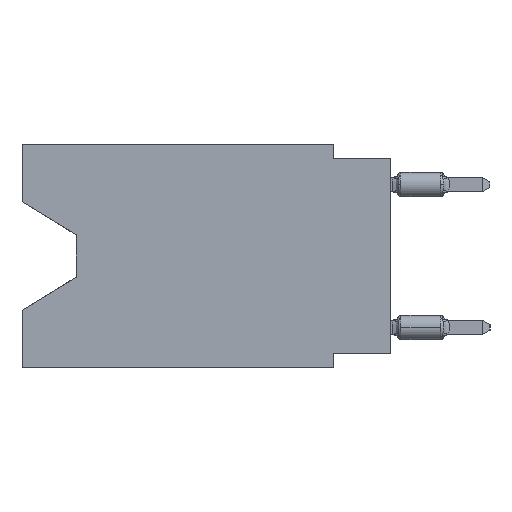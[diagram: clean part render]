
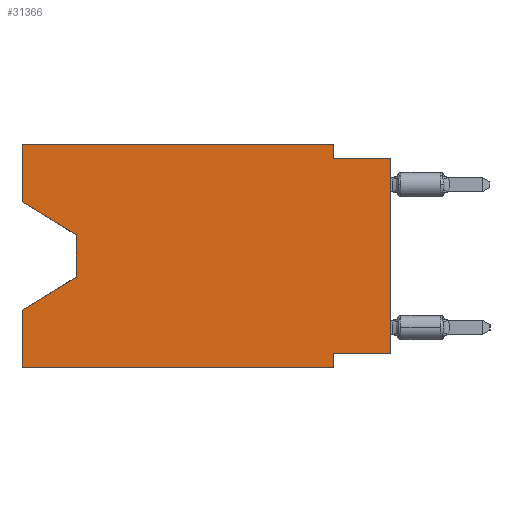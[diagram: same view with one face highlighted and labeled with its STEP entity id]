
A CAD part, left-side view. The second image highlights one B-rep face of the part: STEP entity #31366.
In plain terms, the highlighted planar face has unit normal (-1, 0, 0).
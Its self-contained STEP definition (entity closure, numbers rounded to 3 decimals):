
#161 = VECTOR ( 'NONE', #16425, 1000. ) ;
#222 = DIRECTION ( 'NONE',  ( 0., -1., 0. ) ) ;
#877 = DIRECTION ( 'NONE',  ( 1., 0., 0. ) ) ;
#1106 = CARTESIAN_POINT ( 'NONE',  ( 0., 0., 0. ) ) ;
#1310 = FACE_OUTER_BOUND ( 'NONE', #26498, .T. ) ;
#3058 = EDGE_CURVE ( 'NONE', #6481, #8237, #25895, .T. ) ;
#4183 = DIRECTION ( 'NONE',  ( 0., -1., 0. ) ) ;
#5166 = VERTEX_POINT ( 'NONE', #12029 ) ;
#5691 = EDGE_CURVE ( 'NONE', #41053, #5166, #32945, .T. ) ;
#6027 = CARTESIAN_POINT ( 'NONE',  ( 0., 0., -9.271 ) ) ;
#6143 = CARTESIAN_POINT ( 'NONE',  ( 0., 13.97, -4.013 ) ) ;
#6481 = VERTEX_POINT ( 'NONE', #13730 ) ;
#6867 = LINE ( 'NONE', #6027, #29017 ) ;
#7112 = ORIENTED_EDGE ( 'NONE', *, *, #29976, .F. ) ;
#7142 = VECTOR ( 'NONE', #25878, 1000. ) ;
#7175 = LINE ( 'NONE', #42387, #161 ) ;
#7408 = EDGE_CURVE ( 'NONE', #25848, #33804, #36129, .T. ) ;
#8237 = VERTEX_POINT ( 'NONE', #36243 ) ;
#8855 = ORIENTED_EDGE ( 'NONE', *, *, #14821, .T. ) ;
#8907 = VERTEX_POINT ( 'NONE', #16260 ) ;
#9576 = CARTESIAN_POINT ( 'NONE',  ( 0., 16.383, 0. ) ) ;
#9677 = CARTESIAN_POINT ( 'NONE',  ( 0., 2.54, -9.906 ) ) ;
#9739 = VECTOR ( 'NONE', #33322, 1000. ) ;
#9964 = CARTESIAN_POINT ( 'NONE',  ( 0., 16.383, -9.906 ) ) ;
#10589 = LINE ( 'NONE', #9964, #27923 ) ;
#11843 = DIRECTION ( 'NONE',  ( 0., -0.855, -0.519 ) ) ;
#11880 = CARTESIAN_POINT ( 'NONE',  ( 0., 13.97, -4.013 ) ) ;
#12029 = CARTESIAN_POINT ( 'NONE',  ( 0., 0., -0.635 ) ) ;
#12942 = VECTOR ( 'NONE', #4183, 1000. ) ;
#13730 = CARTESIAN_POINT ( 'NONE',  ( 0., 16.383, -2.546 ) ) ;
#14215 = CARTESIAN_POINT ( 'NONE',  ( 0., 16.383, 0. ) ) ;
#14732 = VECTOR ( 'NONE', #27727, 1000. ) ;
#14821 = EDGE_CURVE ( 'NONE', #28317, #25848, #39166, .T. ) ;
#15124 = ORIENTED_EDGE ( 'NONE', *, *, #39333, .T. ) ;
#15166 = VERTEX_POINT ( 'NONE', #32851 ) ;
#15211 = VERTEX_POINT ( 'NONE', #23599 ) ;
#16260 = CARTESIAN_POINT ( 'NONE',  ( 0., 16.383, -9.906 ) ) ;
#16425 = DIRECTION ( 'NONE',  ( 0., 0., -1. ) ) ;
#17313 = VECTOR ( 'NONE', #20436, 1000. ) ;
#18347 = ORIENTED_EDGE ( 'NONE', *, *, #3058, .F. ) ;
#18407 = DIRECTION ( 'NONE',  ( 0., 0., 1. ) ) ;
#19777 = EDGE_CURVE ( 'NONE', #8237, #15166, #39062, .T. ) ;
#20436 = DIRECTION ( 'NONE',  ( 0., 0., 1. ) ) ;
#20486 = CARTESIAN_POINT ( 'NONE',  ( 0., 13.97, -5.893 ) ) ;
#22194 = EDGE_CURVE ( 'NONE', #15166, #41053, #7175, .T. ) ;
#22539 = DIRECTION ( 'NONE',  ( 0., 1., 0. ) ) ;
#22739 = EDGE_CURVE ( 'NONE', #15211, #5166, #39941, .T. ) ;
#23109 = EDGE_CURVE ( 'NONE', #15211, #31234, #6867, .T. ) ;
#23220 = CARTESIAN_POINT ( 'NONE',  ( 0., 2.54, -9.271 ) ) ;
#23599 = CARTESIAN_POINT ( 'NONE',  ( 0., 0., -9.271 ) ) ;
#23686 = DIRECTION ( 'NONE',  ( 0., -1., 0. ) ) ;
#24348 = ORIENTED_EDGE ( 'NONE', *, *, #19777, .F. ) ;
#24718 = CARTESIAN_POINT ( 'NONE',  ( 0., 16.383, -7.36 ) ) ;
#25225 = VECTOR ( 'NONE', #18407, 1000. ) ;
#25848 = VERTEX_POINT ( 'NONE', #20486 ) ;
#25878 = DIRECTION ( 'NONE',  ( 0., 0., -1. ) ) ;
#25895 = LINE ( 'NONE', #9576, #25225 ) ;
#26426 = DIRECTION ( 'NONE',  ( 0., 0., -1. ) ) ;
#26498 = EDGE_LOOP ( 'NONE', ( #40503, #8855, #33705, #34327, #15124, #7112, #34986, #35897, #36806, #36708, #24348, #18347 ) ) ;
#27484 = CARTESIAN_POINT ( 'NONE',  ( 0., 16.383, 0. ) ) ;
#27727 = DIRECTION ( 'NONE',  ( 0., 0., 1. ) ) ;
#27824 = VECTOR ( 'NONE', #11843, 1000. ) ;
#27923 = VECTOR ( 'NONE', #23686, 1000. ) ;
#28317 = VERTEX_POINT ( 'NONE', #11880 ) ;
#28501 = EDGE_CURVE ( 'NONE', #8907, #33804, #37612, .T. ) ;
#28790 = LINE ( 'NONE', #35214, #27824 ) ;
#29017 = VECTOR ( 'NONE', #22539, 1000. ) ;
#29836 = EDGE_CURVE ( 'NONE', #6481, #28317, #28790, .T. ) ;
#29849 = LINE ( 'NONE', #9677, #37438 ) ;
#29976 = EDGE_CURVE ( 'NONE', #31234, #32635, #29849, .T. ) ;
#30319 = CARTESIAN_POINT ( 'NONE',  ( 0., 13.97, -5.893 ) ) ;
#31234 = VERTEX_POINT ( 'NONE', #23220 ) ;
#31366 = ADVANCED_FACE ( 'NONE', ( #1310 ), #33911, .F. ) ;
#32627 = CARTESIAN_POINT ( 'NONE',  ( 0., 16.383, 0. ) ) ;
#32635 = VERTEX_POINT ( 'NONE', #35578 ) ;
#32739 = CARTESIAN_POINT ( 'NONE',  ( 0., 0., -0.635 ) ) ;
#32851 = CARTESIAN_POINT ( 'NONE',  ( 0., 2.54, 0. ) ) ;
#32945 = LINE ( 'NONE', #32739, #12942 ) ;
#33322 = DIRECTION ( 'NONE',  ( 0., 0.855, -0.519 ) ) ;
#33705 = ORIENTED_EDGE ( 'NONE', *, *, #7408, .T. ) ;
#33804 = VERTEX_POINT ( 'NONE', #24718 ) ;
#33911 = PLANE ( 'NONE',  #41595 ) ;
#34327 = ORIENTED_EDGE ( 'NONE', *, *, #28501, .F. ) ;
#34986 = ORIENTED_EDGE ( 'NONE', *, *, #23109, .F. ) ;
#35214 = CARTESIAN_POINT ( 'NONE',  ( 0., 16.383, -2.546 ) ) ;
#35578 = CARTESIAN_POINT ( 'NONE',  ( 0., 2.54, -9.906 ) ) ;
#35897 = ORIENTED_EDGE ( 'NONE', *, *, #22739, .T. ) ;
#36088 = VECTOR ( 'NONE', #222, 1000. ) ;
#36129 = LINE ( 'NONE', #30319, #9739 ) ;
#36243 = CARTESIAN_POINT ( 'NONE',  ( 0., 16.383, 0. ) ) ;
#36708 = ORIENTED_EDGE ( 'NONE', *, *, #22194, .F. ) ;
#36806 = ORIENTED_EDGE ( 'NONE', *, *, #5691, .F. ) ;
#37438 = VECTOR ( 'NONE', #26426, 1000. ) ;
#37612 = LINE ( 'NONE', #14215, #14732 ) ;
#38502 = CARTESIAN_POINT ( 'NONE',  ( 0., 2.54, -0.635 ) ) ;
#39062 = LINE ( 'NONE', #32627, #36088 ) ;
#39166 = LINE ( 'NONE', #6143, #7142 ) ;
#39333 = EDGE_CURVE ( 'NONE', #8907, #32635, #10589, .T. ) ;
#39941 = LINE ( 'NONE', #1106, #17313 ) ;
#40503 = ORIENTED_EDGE ( 'NONE', *, *, #29836, .T. ) ;
#40566 = DIRECTION ( 'NONE',  ( 0., 0., -1. ) ) ;
#41053 = VERTEX_POINT ( 'NONE', #38502 ) ;
#41595 = AXIS2_PLACEMENT_3D ( 'NONE', #27484, #877, #40566 ) ;
#42387 = CARTESIAN_POINT ( 'NONE',  ( 0., 2.54, 0. ) ) ;
